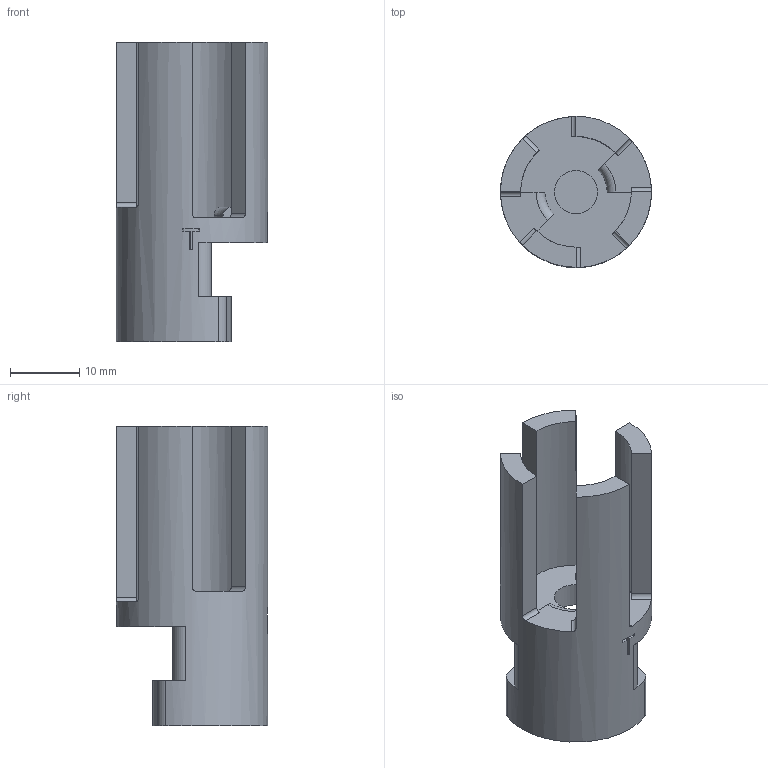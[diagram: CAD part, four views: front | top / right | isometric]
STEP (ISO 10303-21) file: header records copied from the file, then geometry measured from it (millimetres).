
FILE_DESCRIPTION(/* description */ (''),/* implementation_level */ '2;1');
FILE_NAME(/* name */ 'Throating End Pilot Metric (6mm).stp',/* time_stamp */ '2021-02-15T01:39:06-06:00',/* author */ ('johne'),/* organization */ (''),/* preprocessor_version */ 'ST-DEVELOPER v18',/* originating_system */ 'Autodesk Inventor 2020',/* authorisation */ '');
FILE_SCHEMA (('AUTOMOTIVE_DESIGN { 1 0 10303 214 3 1 1 }'));
Length unit declared in the file: millimetre
Products named in the file (1): Throating Tool 6mm rod
Bounding box: 21.84 x 21.84 x 43.36 mm (x, y, z)
Volume: 5757.1 mm3; surface area: 4055.8 mm2
Topology: 1 solids, 1 shells, 55 faces, 160 edges, 113 vertices
Faces by surface type: plane 31, cylinder 22, torus 2
Full cylindrical faces by diameter (mm): 6.25 x1, 21.844 x1
Entity records: 1989 total; most frequent: CARTESIAN_POINT 468, ORIENTED_EDGE 310, DIRECTION 306, EDGE_CURVE 155, AXIS2_PLACEMENT_3D 111, VERTEX_POINT 103, LINE 84, VECTOR 84
